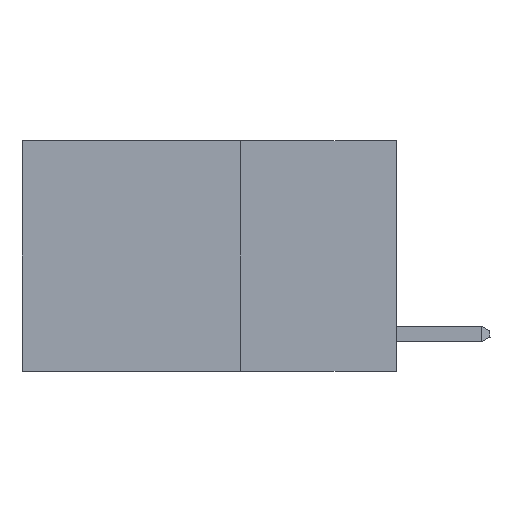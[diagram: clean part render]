
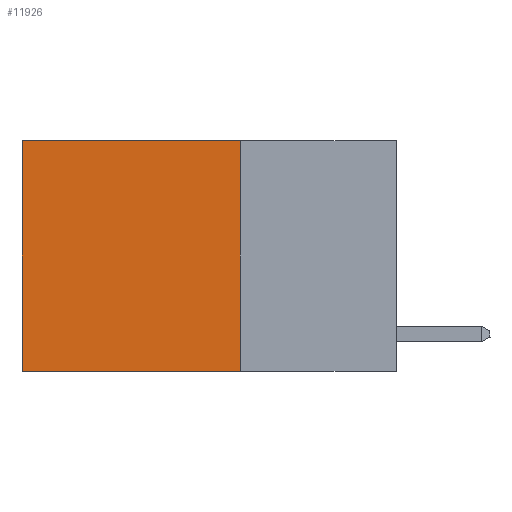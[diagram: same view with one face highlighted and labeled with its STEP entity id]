
A CAD part, left-side view. The second image highlights one B-rep face of the part: STEP entity #11926.
In plain terms, the highlighted planar face has unit normal (-1, 0, 0).
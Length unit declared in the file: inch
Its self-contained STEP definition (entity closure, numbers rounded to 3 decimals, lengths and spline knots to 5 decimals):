
#1332 = VERTEX_POINT ( 'NONE', #2403 ) ;
#2019 = LINE ( 'NONE', #5961, #9993 ) ;
#2182 = VERTEX_POINT ( 'NONE', #20096 ) ;
#2403 = CARTESIAN_POINT ( 'NONE',  ( 0.2625, 0.25, 0. ) ) ;
#2624 = CARTESIAN_POINT ( 'NONE',  ( 0.2625, 0.25, -0.37 ) ) ;
#3725 = EDGE_LOOP ( 'NONE', ( #12399, #3740, #20069, #16576 ) ) ;
#3740 = ORIENTED_EDGE ( 'NONE', *, *, #9358, .F. ) ;
#4240 = DIRECTION ( 'NONE',  ( 0., 1., 0. ) ) ;
#4720 = DIRECTION ( 'NONE',  ( 0., 0., -1. ) ) ;
#5961 = CARTESIAN_POINT ( 'NONE',  ( 0.2625, 0.25, 0. ) ) ;
#7811 = EDGE_CURVE ( 'NONE', #1332, #20471, #13433, .T. ) ;
#8195 = AXIS2_PLACEMENT_3D ( 'NONE', #8851, #19828, #10445 ) ;
#8680 = DIRECTION ( 'NONE',  ( 0., 1., 0. ) ) ;
#8851 = CARTESIAN_POINT ( 'NONE',  ( 0.2625, 0.25, 0. ) ) ;
#9358 = EDGE_CURVE ( 'NONE', #20471, #2182, #9959, .T. ) ;
#9556 = EDGE_CURVE ( 'NONE', #17530, #2182, #18023, .T. ) ;
#9693 = VECTOR ( 'NONE', #4720, 39.37008 ) ;
#9781 = VECTOR ( 'NONE', #18211, 39.37008 ) ;
#9959 = LINE ( 'NONE', #2624, #17792 ) ;
#9993 = VECTOR ( 'NONE', #8680, 39.37008 ) ;
#10445 = DIRECTION ( 'NONE',  ( 0., 0., -1. ) ) ;
#10560 = CARTESIAN_POINT ( 'NONE',  ( 0.2625, 0.6, 0. ) ) ;
#11926 = ADVANCED_FACE ( 'NONE', ( #18442 ), #18243, .F. ) ;
#12399 = ORIENTED_EDGE ( 'NONE', *, *, #9556, .T. ) ;
#13433 = LINE ( 'NONE', #16697, #9781 ) ;
#15707 = CARTESIAN_POINT ( 'NONE',  ( 0.2625, 0.6, 0. ) ) ;
#16576 = ORIENTED_EDGE ( 'NONE', *, *, #18230, .T. ) ;
#16697 = CARTESIAN_POINT ( 'NONE',  ( 0.2625, 0.25, 0. ) ) ;
#17530 = VERTEX_POINT ( 'NONE', #10560 ) ;
#17792 = VECTOR ( 'NONE', #4240, 39.37008 ) ;
#18023 = LINE ( 'NONE', #15707, #9693 ) ;
#18211 = DIRECTION ( 'NONE',  ( 0., 0., -1. ) ) ;
#18230 = EDGE_CURVE ( 'NONE', #1332, #17530, #2019, .T. ) ;
#18243 = PLANE ( 'NONE',  #8195 ) ;
#18442 = FACE_OUTER_BOUND ( 'NONE', #3725, .T. ) ;
#19828 = DIRECTION ( 'NONE',  ( 1., 0., 0. ) ) ;
#20069 = ORIENTED_EDGE ( 'NONE', *, *, #7811, .F. ) ;
#20096 = CARTESIAN_POINT ( 'NONE',  ( 0.2625, 0.6, -0.37 ) ) ;
#20466 = CARTESIAN_POINT ( 'NONE',  ( 0.2625, 0.25, -0.37 ) ) ;
#20471 = VERTEX_POINT ( 'NONE', #20466 ) ;
